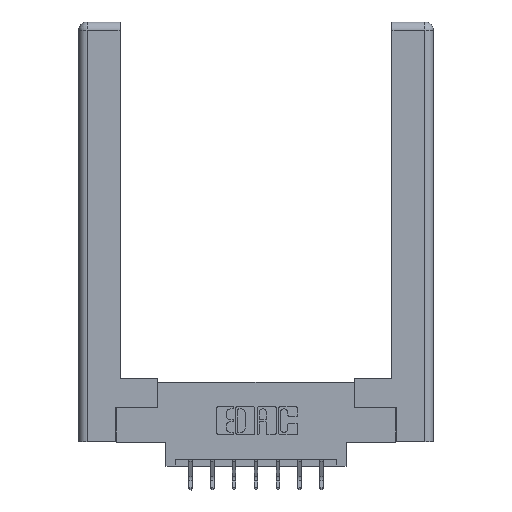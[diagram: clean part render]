
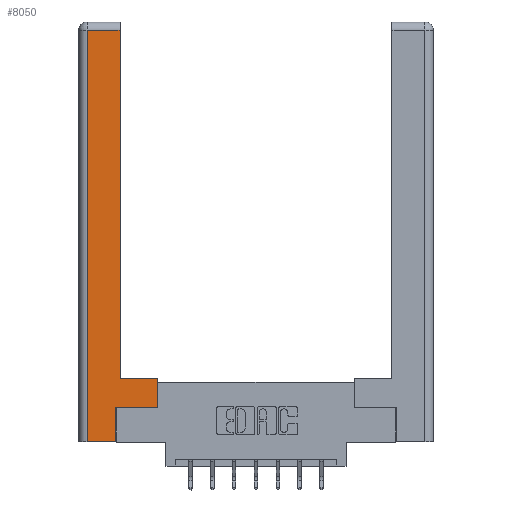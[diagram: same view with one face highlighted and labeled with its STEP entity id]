
A CAD part, top view. The second image highlights one B-rep face of the part: STEP entity #8050.
In plain terms, the highlighted planar face has unit normal (0, 0, 1).
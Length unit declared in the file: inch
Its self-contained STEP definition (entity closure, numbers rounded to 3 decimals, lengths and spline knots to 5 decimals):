
#144 = ORIENTED_EDGE ( 'NONE', *, *, #2988, .T. ) ;
#283 = LINE ( 'NONE', #6012, #3080 ) ;
#322 = LINE ( 'NONE', #11729, #465 ) ;
#465 = VECTOR ( 'NONE', #3613, 39.37008 ) ;
#999 = DIRECTION ( 'NONE',  ( -1., 0., 0. ) ) ;
#1009 = VECTOR ( 'NONE', #10127, 39.37008 ) ;
#1251 = ORIENTED_EDGE ( 'NONE', *, *, #7600, .T. ) ;
#1533 = LINE ( 'NONE', #1982, #1670 ) ;
#1670 = VECTOR ( 'NONE', #7122, 39.37008 ) ;
#1982 = CARTESIAN_POINT ( 'NONE',  ( 0.565, 0.245, 0. ) ) ;
#2058 = DIRECTION ( 'NONE',  ( -1., 0., 0. ) ) ;
#2073 = LINE ( 'NONE', #3072, #10832 ) ;
#2435 = ORIENTED_EDGE ( 'NONE', *, *, #7745, .T. ) ;
#2619 = CARTESIAN_POINT ( 'NONE',  ( 0.0615, 0., 0. ) ) ;
#2988 = EDGE_CURVE ( 'NONE', #9242, #6999, #9164, .T. ) ;
#3072 = CARTESIAN_POINT ( 'NONE',  ( 0.0615, 2.94, 0. ) ) ;
#3080 = VECTOR ( 'NONE', #3108, 39.37008 ) ;
#3108 = DIRECTION ( 'NONE',  ( 0., 1., 0. ) ) ;
#3280 = ORIENTED_EDGE ( 'NONE', *, *, #12926, .T. ) ;
#3432 = VERTEX_POINT ( 'NONE', #8398 ) ;
#3613 = DIRECTION ( 'NONE',  ( 0., 1., 0. ) ) ;
#3965 = CARTESIAN_POINT ( 'NONE',  ( 0.295, 0.45, 0. ) ) ;
#3968 = CARTESIAN_POINT ( 'NONE',  ( 0.265, 0., 0. ) ) ;
#4097 = EDGE_LOOP ( 'NONE', ( #144, #3280, #10020, #9579, #9389, #2435, #1251, #10362 ) ) ;
#4360 = FACE_OUTER_BOUND ( 'NONE', #4097, .T. ) ;
#4742 = CARTESIAN_POINT ( 'NONE',  ( 0.265, 0.245, 0. ) ) ;
#4920 = VERTEX_POINT ( 'NONE', #3968 ) ;
#4967 = DIRECTION ( 'NONE',  ( 0., 0., -1. ) ) ;
#4996 = EDGE_CURVE ( 'NONE', #10937, #9452, #10830, .T. ) ;
#5008 = DIRECTION ( 'NONE',  ( -1., 0., 0. ) ) ;
#5295 = VERTEX_POINT ( 'NONE', #4742 ) ;
#5932 = EDGE_CURVE ( 'NONE', #9452, #4920, #9255, .T. ) ;
#6012 = CARTESIAN_POINT ( 'NONE',  ( 0.265, 0.245, 0. ) ) ;
#6107 = CARTESIAN_POINT ( 'NONE',  ( 0.0615, 0., 0. ) ) ;
#6596 = VECTOR ( 'NONE', #11909, 39.37008 ) ;
#6933 = CARTESIAN_POINT ( 'NONE',  ( 0., 0., 0. ) ) ;
#6999 = VERTEX_POINT ( 'NONE', #7676 ) ;
#7031 = DIRECTION ( 'NONE',  ( 0., -1., 0. ) ) ;
#7122 = DIRECTION ( 'NONE',  ( 1., 0., 0. ) ) ;
#7353 = AXIS2_PLACEMENT_3D ( 'NONE', #6933, #4967, #5008 ) ;
#7600 = EDGE_CURVE ( 'NONE', #3432, #8741, #322, .T. ) ;
#7676 = CARTESIAN_POINT ( 'NONE',  ( 0.295, 2.94, 0. ) ) ;
#7745 = EDGE_CURVE ( 'NONE', #5295, #3432, #1533, .T. ) ;
#7865 = CARTESIAN_POINT ( 'NONE',  ( 0.295, 3., 0. ) ) ;
#7894 = CARTESIAN_POINT ( 'NONE',  ( 0.0615, 2.94, 0. ) ) ;
#8050 = ADVANCED_FACE ( 'NONE', ( #4360 ), #10895, .F. ) ;
#8398 = CARTESIAN_POINT ( 'NONE',  ( 0.565, 0.245, 0. ) ) ;
#8741 = VERTEX_POINT ( 'NONE', #9707 ) ;
#8944 = EDGE_CURVE ( 'NONE', #8741, #9242, #11066, .T. ) ;
#8978 = EDGE_CURVE ( 'NONE', #4920, #5295, #283, .T. ) ;
#9164 = LINE ( 'NONE', #7865, #1009 ) ;
#9242 = VERTEX_POINT ( 'NONE', #10735 ) ;
#9255 = LINE ( 'NONE', #11038, #6596 ) ;
#9389 = ORIENTED_EDGE ( 'NONE', *, *, #8978, .T. ) ;
#9452 = VERTEX_POINT ( 'NONE', #2619 ) ;
#9579 = ORIENTED_EDGE ( 'NONE', *, *, #5932, .T. ) ;
#9707 = CARTESIAN_POINT ( 'NONE',  ( 0.565, 0.45, 0. ) ) ;
#10020 = ORIENTED_EDGE ( 'NONE', *, *, #4996, .T. ) ;
#10127 = DIRECTION ( 'NONE',  ( 0., 1., 0. ) ) ;
#10362 = ORIENTED_EDGE ( 'NONE', *, *, #8944, .T. ) ;
#10681 = VECTOR ( 'NONE', #7031, 39.37008 ) ;
#10735 = CARTESIAN_POINT ( 'NONE',  ( 0.295, 0.45, 0. ) ) ;
#10830 = LINE ( 'NONE', #6107, #10681 ) ;
#10832 = VECTOR ( 'NONE', #2058, 39.37008 ) ;
#10895 = PLANE ( 'NONE',  #7353 ) ;
#10937 = VERTEX_POINT ( 'NONE', #7894 ) ;
#11038 = CARTESIAN_POINT ( 'NONE',  ( 0.265, 0., 0. ) ) ;
#11066 = LINE ( 'NONE', #3965, #11997 ) ;
#11729 = CARTESIAN_POINT ( 'NONE',  ( 0.565, 0.45, 0. ) ) ;
#11909 = DIRECTION ( 'NONE',  ( 1., 0., 0. ) ) ;
#11997 = VECTOR ( 'NONE', #999, 39.37008 ) ;
#12926 = EDGE_CURVE ( 'NONE', #6999, #10937, #2073, .T. ) ;
